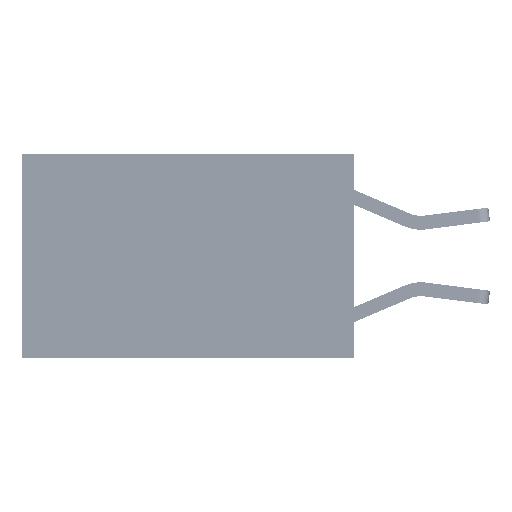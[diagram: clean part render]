
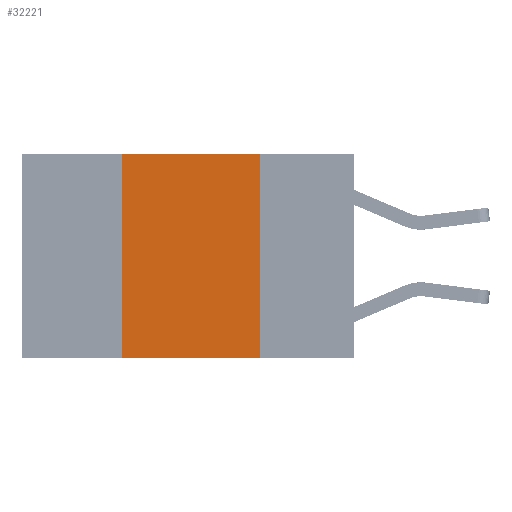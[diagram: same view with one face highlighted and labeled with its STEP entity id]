
A CAD part, left-side view. The second image highlights one B-rep face of the part: STEP entity #32221.
In plain terms, the highlighted planar face has unit normal (-1, 0, 0).
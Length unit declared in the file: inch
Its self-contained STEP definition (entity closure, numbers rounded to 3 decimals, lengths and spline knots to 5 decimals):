
#2673 = VERTEX_POINT ( 'NONE', #23317 ) ;
#2819 = CARTESIAN_POINT ( 'NONE',  ( 0., 0.17, -0.37 ) ) ;
#2977 = CARTESIAN_POINT ( 'NONE',  ( 0., 0.42, -0.37 ) ) ;
#3390 = EDGE_CURVE ( 'NONE', #2673, #3636, #31349, .T. ) ;
#3636 = VERTEX_POINT ( 'NONE', #29954 ) ;
#5908 = VECTOR ( 'NONE', #11384, 39.37008 ) ;
#8517 = VECTOR ( 'NONE', #31014, 39.37008 ) ;
#9309 = VECTOR ( 'NONE', #28444, 39.37008 ) ;
#9849 = EDGE_CURVE ( 'NONE', #11020, #2673, #31917, .T. ) ;
#10102 = CARTESIAN_POINT ( 'NONE',  ( 0., 0.17, 0. ) ) ;
#11020 = VERTEX_POINT ( 'NONE', #2977 ) ;
#11384 = DIRECTION ( 'NONE',  ( 0., -1., 0. ) ) ;
#13856 = VERTEX_POINT ( 'NONE', #2819 ) ;
#14064 = EDGE_CURVE ( 'NONE', #11020, #13856, #19320, .T. ) ;
#14225 = CARTESIAN_POINT ( 'NONE',  ( 0., 0.42, 0. ) ) ;
#14408 = AXIS2_PLACEMENT_3D ( 'NONE', #25265, #17871, #22719 ) ;
#16587 = DIRECTION ( 'NONE',  ( 0., 0., 1. ) ) ;
#17871 = DIRECTION ( 'NONE',  ( 1., 0., 0. ) ) ;
#18039 = FACE_OUTER_BOUND ( 'NONE', #32229, .T. ) ;
#19320 = LINE ( 'NONE', #21988, #5908 ) ;
#21277 = ORIENTED_EDGE ( 'NONE', *, *, #14064, .T. ) ;
#21988 = CARTESIAN_POINT ( 'NONE',  ( 0., 0.6, -0.37 ) ) ;
#22719 = DIRECTION ( 'NONE',  ( 0., 0., -1. ) ) ;
#23317 = CARTESIAN_POINT ( 'NONE',  ( 0., 0.42, 0. ) ) ;
#25265 = CARTESIAN_POINT ( 'NONE',  ( 0., 0.6, 0. ) ) ;
#25798 = CARTESIAN_POINT ( 'NONE',  ( 0., 0.6, 0. ) ) ;
#27337 = ORIENTED_EDGE ( 'NONE', *, *, #3390, .F. ) ;
#28075 = EDGE_CURVE ( 'NONE', #3636, #13856, #30987, .T. ) ;
#28444 = DIRECTION ( 'NONE',  ( 0., 0., -1. ) ) ;
#28652 = ORIENTED_EDGE ( 'NONE', *, *, #28075, .F. ) ;
#29954 = CARTESIAN_POINT ( 'NONE',  ( 0., 0.17, 0. ) ) ;
#30826 = PLANE ( 'NONE',  #14408 ) ;
#30987 = LINE ( 'NONE', #10102, #9309 ) ;
#31014 = DIRECTION ( 'NONE',  ( 0., -1., 0. ) ) ;
#31259 = VECTOR ( 'NONE', #16587, 39.37008 ) ;
#31349 = LINE ( 'NONE', #25798, #8517 ) ;
#31917 = LINE ( 'NONE', #14225, #31259 ) ;
#32162 = ORIENTED_EDGE ( 'NONE', *, *, #9849, .F. ) ;
#32221 = ADVANCED_FACE ( 'NONE', ( #18039 ), #30826, .F. ) ;
#32229 = EDGE_LOOP ( 'NONE', ( #28652, #27337, #32162, #21277 ) ) ;
